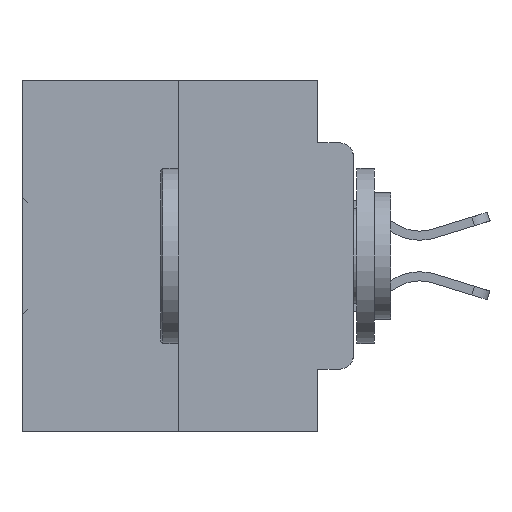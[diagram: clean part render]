
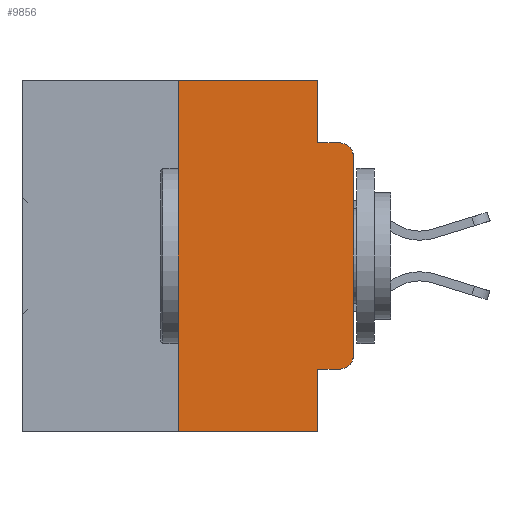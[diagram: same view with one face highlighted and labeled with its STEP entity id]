
A CAD part, left-side view. The second image highlights one B-rep face of the part: STEP entity #9856.
In plain terms, the highlighted planar face has unit normal (-1, 0, 0).
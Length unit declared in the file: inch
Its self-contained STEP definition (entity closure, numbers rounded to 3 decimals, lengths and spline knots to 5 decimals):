
#80 = EDGE_CURVE ( 'NONE', #2416, #8197, #14162, .T. ) ;
#213 = LINE ( 'NONE', #21330, #8604 ) ;
#966 = ORIENTED_EDGE ( 'NONE', *, *, #31894, .T. ) ;
#1035 = LINE ( 'NONE', #11205, #15947 ) ;
#1371 = FACE_OUTER_BOUND ( 'NONE', #32628, .T. ) ;
#1428 = VECTOR ( 'NONE', #24610, 39.37008 ) ;
#1883 = CARTESIAN_POINT ( 'NONE',  ( 0., 0.02, -0.1085 ) ) ;
#2265 = CIRCLE ( 'NONE', #23647, 0.02 ) ;
#2267 = ORIENTED_EDGE ( 'NONE', *, *, #26508, .F. ) ;
#2416 = VERTEX_POINT ( 'NONE', #33673 ) ;
#3658 = DIRECTION ( 'NONE',  ( 0., -1., 0. ) ) ;
#3932 = CARTESIAN_POINT ( 'NONE',  ( 0., 0.02, -0.0885 ) ) ;
#4496 = DIRECTION ( 'NONE',  ( 1., 0., 0. ) ) ;
#4638 = LINE ( 'NONE', #31881, #19540 ) ;
#4684 = DIRECTION ( 'NONE',  ( 0., 0., -1. ) ) ;
#5143 = DIRECTION ( 'NONE',  ( 0., -1., 0. ) ) ;
#5198 = DIRECTION ( 'NONE',  ( 0., -1., 0. ) ) ;
#5777 = ORIENTED_EDGE ( 'NONE', *, *, #22843, .F. ) ;
#5989 = CIRCLE ( 'NONE', #8418, 0.02 ) ;
#6178 = VERTEX_POINT ( 'NONE', #24130 ) ;
#6241 = CARTESIAN_POINT ( 'NONE',  ( 0., 0.02, -0.3915 ) ) ;
#7136 = ORIENTED_EDGE ( 'NONE', *, *, #27194, .T. ) ;
#7251 = EDGE_CURVE ( 'NONE', #20862, #25308, #4638, .T. ) ;
#7433 = DIRECTION ( 'NONE',  ( 0., -1., 0. ) ) ;
#7449 = CARTESIAN_POINT ( 'NONE',  ( 0., 0.051, 0. ) ) ;
#7971 = EDGE_CURVE ( 'NONE', #28409, #23369, #10807, .T. ) ;
#8006 = ORIENTED_EDGE ( 'NONE', *, *, #32029, .F. ) ;
#8037 = CARTESIAN_POINT ( 'NONE',  ( 0., 0.25, 0. ) ) ;
#8197 = VERTEX_POINT ( 'NONE', #27659 ) ;
#8291 = CARTESIAN_POINT ( 'NONE',  ( 0., 0.051, 0. ) ) ;
#8418 = AXIS2_PLACEMENT_3D ( 'NONE', #6241, #25662, #9116 ) ;
#8604 = VECTOR ( 'NONE', #7433, 39.37008 ) ;
#8928 = CARTESIAN_POINT ( 'NONE',  ( 0., 0.051, -0.4115 ) ) ;
#9034 = VECTOR ( 'NONE', #5198, 39.37008 ) ;
#9116 = DIRECTION ( 'NONE',  ( 0., 0., -1. ) ) ;
#9134 = CARTESIAN_POINT ( 'NONE',  ( 0., 0.02, -0.4115 ) ) ;
#9856 = ADVANCED_FACE ( 'NONE', ( #1371 ), #32113, .F. ) ;
#9918 = LINE ( 'NONE', #30169, #9034 ) ;
#10807 = LINE ( 'NONE', #7449, #24593 ) ;
#11092 = ORIENTED_EDGE ( 'NONE', *, *, #7251, .T. ) ;
#11102 = VERTEX_POINT ( 'NONE', #9134 ) ;
#11128 = ORIENTED_EDGE ( 'NONE', *, *, #7971, .F. ) ;
#11205 = CARTESIAN_POINT ( 'NONE',  ( 0., 0.051, -0.4115 ) ) ;
#11440 = CARTESIAN_POINT ( 'NONE',  ( 0., 0., -0.1085 ) ) ;
#12623 = DIRECTION ( 'NONE',  ( 0., 0., 1. ) ) ;
#12814 = ORIENTED_EDGE ( 'NONE', *, *, #33806, .T. ) ;
#14162 = LINE ( 'NONE', #29237, #35133 ) ;
#15827 = VERTEX_POINT ( 'NONE', #3932 ) ;
#15947 = VECTOR ( 'NONE', #3658, 39.37008 ) ;
#19540 = VECTOR ( 'NONE', #12623, 39.37008 ) ;
#20862 = VERTEX_POINT ( 'NONE', #32265 ) ;
#21238 = CARTESIAN_POINT ( 'NONE',  ( 0., 0.473, 0. ) ) ;
#21330 = CARTESIAN_POINT ( 'NONE',  ( 0., 0.473, -0.5 ) ) ;
#21344 = LINE ( 'NONE', #8291, #35807 ) ;
#21428 = DIRECTION ( 'NONE',  ( -1., 0., 0. ) ) ;
#22807 = LINE ( 'NONE', #8037, #1428 ) ;
#22843 = EDGE_CURVE ( 'NONE', #6178, #2416, #22807, .T. ) ;
#23369 = VERTEX_POINT ( 'NONE', #24466 ) ;
#23647 = AXIS2_PLACEMENT_3D ( 'NONE', #1883, #21428, #4684 ) ;
#23955 = DIRECTION ( 'NONE',  ( 0., 0., -1. ) ) ;
#24130 = CARTESIAN_POINT ( 'NONE',  ( 0., 0.25, -0.5 ) ) ;
#24466 = CARTESIAN_POINT ( 'NONE',  ( 0., 0.051, -0.5 ) ) ;
#24593 = VECTOR ( 'NONE', #26817, 39.37008 ) ;
#24610 = DIRECTION ( 'NONE',  ( 0., 0., 1. ) ) ;
#25308 = VERTEX_POINT ( 'NONE', #11440 ) ;
#25328 = ORIENTED_EDGE ( 'NONE', *, *, #80, .F. ) ;
#25635 = AXIS2_PLACEMENT_3D ( 'NONE', #21238, #4496, #23955 ) ;
#25662 = DIRECTION ( 'NONE',  ( -1., 0., 0. ) ) ;
#26508 = EDGE_CURVE ( 'NONE', #8197, #30173, #21344, .T. ) ;
#26638 = ORIENTED_EDGE ( 'NONE', *, *, #32678, .T. ) ;
#26817 = DIRECTION ( 'NONE',  ( 0., 0., -1. ) ) ;
#27194 = EDGE_CURVE ( 'NONE', #11102, #20862, #5989, .T. ) ;
#27620 = DIRECTION ( 'NONE',  ( 0., 0., -1. ) ) ;
#27639 = CARTESIAN_POINT ( 'NONE',  ( 0., 0.051, -0.0885 ) ) ;
#27659 = CARTESIAN_POINT ( 'NONE',  ( 0., 0.051, 0. ) ) ;
#28409 = VERTEX_POINT ( 'NONE', #8928 ) ;
#29237 = CARTESIAN_POINT ( 'NONE',  ( 0., 0.473, 0. ) ) ;
#30169 = CARTESIAN_POINT ( 'NONE',  ( 0., 0.051, -0.0885 ) ) ;
#30173 = VERTEX_POINT ( 'NONE', #27639 ) ;
#31881 = CARTESIAN_POINT ( 'NONE',  ( 0., 0., 0. ) ) ;
#31894 = EDGE_CURVE ( 'NONE', #6178, #23369, #213, .T. ) ;
#32029 = EDGE_CURVE ( 'NONE', #30173, #15827, #9918, .T. ) ;
#32113 = PLANE ( 'NONE',  #25635 ) ;
#32265 = CARTESIAN_POINT ( 'NONE',  ( 0., 0., -0.3915 ) ) ;
#32628 = EDGE_LOOP ( 'NONE', ( #11092, #12814, #8006, #2267, #25328, #5777, #966, #11128, #26638, #7136 ) ) ;
#32678 = EDGE_CURVE ( 'NONE', #28409, #11102, #1035, .T. ) ;
#33673 = CARTESIAN_POINT ( 'NONE',  ( 0., 0.25, 0. ) ) ;
#33806 = EDGE_CURVE ( 'NONE', #25308, #15827, #2265, .T. ) ;
#35133 = VECTOR ( 'NONE', #5143, 39.37008 ) ;
#35807 = VECTOR ( 'NONE', #27620, 39.37008 ) ;
